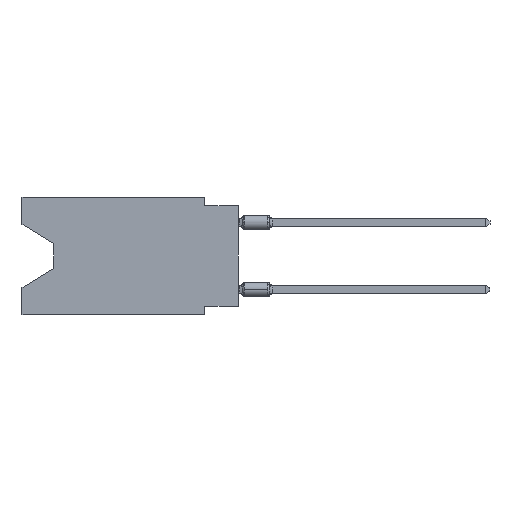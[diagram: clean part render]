
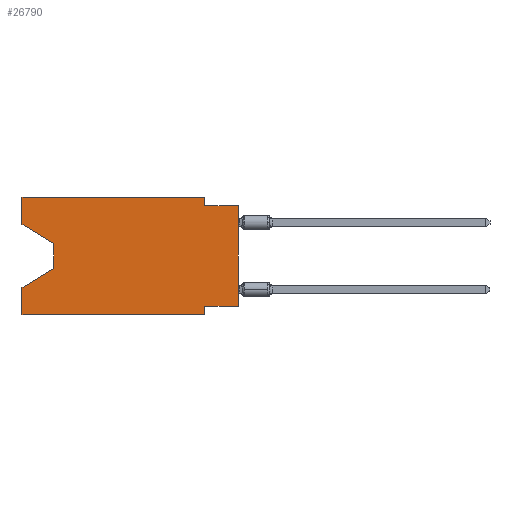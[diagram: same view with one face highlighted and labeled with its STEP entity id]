
A CAD part, left-side view. The second image highlights one B-rep face of the part: STEP entity #26790.
In plain terms, the highlighted planar face has unit normal (-1, 0, 0).
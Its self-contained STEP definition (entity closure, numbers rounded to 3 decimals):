
#3 = VECTOR ( 'NONE', #8153, 1000. ) ;
#32 = DIRECTION ( 'NONE',  ( 0., -1., 0. ) ) ;
#323 = VERTEX_POINT ( 'NONE', #29746 ) ;
#369 = LINE ( 'NONE', #28039, #20729 ) ;
#411 = DIRECTION ( 'NONE',  ( 0., 0., 1. ) ) ;
#494 = VECTOR ( 'NONE', #32, 1000. ) ;
#666 = CARTESIAN_POINT ( 'NONE',  ( 0., 16.383, 0. ) ) ;
#976 = DIRECTION ( 'NONE',  ( 0., 0., 1. ) ) ;
#1653 = EDGE_CURVE ( 'NONE', #4781, #33622, #13022, .T. ) ;
#1705 = VERTEX_POINT ( 'NONE', #1808 ) ;
#1808 = CARTESIAN_POINT ( 'NONE',  ( 0., 16.383, -2.038 ) ) ;
#1922 = VECTOR ( 'NONE', #24212, 1000. ) ;
#2004 = EDGE_CURVE ( 'NONE', #2498, #8590, #10922, .T. ) ;
#2134 = EDGE_CURVE ( 'NONE', #1705, #15088, #6054, .T. ) ;
#2196 = VERTEX_POINT ( 'NONE', #30822 ) ;
#2271 = CARTESIAN_POINT ( 'NONE',  ( 0., 2.54, 0. ) ) ;
#2498 = VERTEX_POINT ( 'NONE', #13072 ) ;
#2718 = CARTESIAN_POINT ( 'NONE',  ( 0., 16.383, -8.89 ) ) ;
#2837 = DIRECTION ( 'NONE',  ( 0., 0., -1. ) ) ;
#2867 = VECTOR ( 'NONE', #18896, 1000. ) ;
#3170 = EDGE_CURVE ( 'NONE', #2196, #8590, #26371, .T. ) ;
#3635 = DIRECTION ( 'NONE',  ( 0., 0., -1. ) ) ;
#3672 = EDGE_CURVE ( 'NONE', #15088, #33728, #13118, .T. ) ;
#3768 = ORIENTED_EDGE ( 'NONE', *, *, #2004, .T. ) ;
#3801 = CARTESIAN_POINT ( 'NONE',  ( 0., 16.383, 0. ) ) ;
#4375 = CARTESIAN_POINT ( 'NONE',  ( 0., 13.97, -3.505 ) ) ;
#4781 = VERTEX_POINT ( 'NONE', #31938 ) ;
#6054 = LINE ( 'NONE', #6597, #19264 ) ;
#6102 = CARTESIAN_POINT ( 'NONE',  ( 0., 2.54, 0. ) ) ;
#6143 = ORIENTED_EDGE ( 'NONE', *, *, #29639, .F. ) ;
#6597 = CARTESIAN_POINT ( 'NONE',  ( 0., 16.383, 0. ) ) ;
#6748 = CARTESIAN_POINT ( 'NONE',  ( 0., 16.383, -6.852 ) ) ;
#6887 = ORIENTED_EDGE ( 'NONE', *, *, #19787, .F. ) ;
#7578 = EDGE_CURVE ( 'NONE', #31840, #2498, #369, .T. ) ;
#7704 = CARTESIAN_POINT ( 'NONE',  ( 0., 16.383, 0. ) ) ;
#7708 = CARTESIAN_POINT ( 'NONE',  ( 0., 0., -8.255 ) ) ;
#7753 = LINE ( 'NONE', #30144, #22326 ) ;
#7934 = ORIENTED_EDGE ( 'NONE', *, *, #1653, .F. ) ;
#8043 = DIRECTION ( 'NONE',  ( 0., 0.855, -0.519 ) ) ;
#8153 = DIRECTION ( 'NONE',  ( 0., -1., 0. ) ) ;
#8253 = ORIENTED_EDGE ( 'NONE', *, *, #31693, .T. ) ;
#8590 = VERTEX_POINT ( 'NONE', #6748 ) ;
#9278 = CARTESIAN_POINT ( 'NONE',  ( 0., 0., 0. ) ) ;
#10867 = EDGE_CURVE ( 'NONE', #20718, #18394, #35172, .T. ) ;
#10922 = LINE ( 'NONE', #27208, #11189 ) ;
#11189 = VECTOR ( 'NONE', #8043, 1000. ) ;
#11339 = PLANE ( 'NONE',  #31923 ) ;
#11459 = VECTOR ( 'NONE', #26016, 1000. ) ;
#13022 = LINE ( 'NONE', #21503, #1922 ) ;
#13072 = CARTESIAN_POINT ( 'NONE',  ( 0., 13.97, -5.385 ) ) ;
#13118 = LINE ( 'NONE', #7704, #494 ) ;
#13483 = ORIENTED_EDGE ( 'NONE', *, *, #24575, .T. ) ;
#14204 = EDGE_CURVE ( 'NONE', #1705, #31840, #7753, .T. ) ;
#14849 = ORIENTED_EDGE ( 'NONE', *, *, #2134, .F. ) ;
#15088 = VERTEX_POINT ( 'NONE', #3801 ) ;
#16767 = FACE_OUTER_BOUND ( 'NONE', #23823, .T. ) ;
#18394 = VERTEX_POINT ( 'NONE', #23117 ) ;
#18756 = ORIENTED_EDGE ( 'NONE', *, *, #3170, .F. ) ;
#18788 = ORIENTED_EDGE ( 'NONE', *, *, #7578, .T. ) ;
#18896 = DIRECTION ( 'NONE',  ( 0., 1., 0. ) ) ;
#19264 = VECTOR ( 'NONE', #976, 1000. ) ;
#19731 = CARTESIAN_POINT ( 'NONE',  ( 0., 2.54, -8.89 ) ) ;
#19787 = EDGE_CURVE ( 'NONE', #18394, #323, #33647, .T. ) ;
#20397 = ORIENTED_EDGE ( 'NONE', *, *, #14204, .T. ) ;
#20718 = VERTEX_POINT ( 'NONE', #35223 ) ;
#20729 = VECTOR ( 'NONE', #22437, 1000. ) ;
#21086 = ORIENTED_EDGE ( 'NONE', *, *, #3672, .F. ) ;
#21503 = CARTESIAN_POINT ( 'NONE',  ( 0., 0., -0.635 ) ) ;
#22326 = VECTOR ( 'NONE', #29792, 1000. ) ;
#22437 = DIRECTION ( 'NONE',  ( 0., 0., -1. ) ) ;
#22557 = DIRECTION ( 'NONE',  ( 1., 0., 0. ) ) ;
#22745 = DIRECTION ( 'NONE',  ( 0., 0., -1. ) ) ;
#22759 = CARTESIAN_POINT ( 'NONE',  ( 0., 0., -0.635 ) ) ;
#22816 = VECTOR ( 'NONE', #22745, 1000. ) ;
#22919 = LINE ( 'NONE', #6102, #22816 ) ;
#23117 = CARTESIAN_POINT ( 'NONE',  ( 0., 2.54, -8.255 ) ) ;
#23823 = EDGE_LOOP ( 'NONE', ( #20397, #18788, #3768, #18756, #13483, #6887, #31657, #8253, #7934, #6143, #21086, #14849 ) ) ;
#24212 = DIRECTION ( 'NONE',  ( 0., -1., 0. ) ) ;
#24575 = EDGE_CURVE ( 'NONE', #2196, #323, #32902, .T. ) ;
#26016 = DIRECTION ( 'NONE',  ( 0., 0., 1. ) ) ;
#26371 = LINE ( 'NONE', #31795, #11459 ) ;
#26790 = ADVANCED_FACE ( 'NONE', ( #16767 ), #11339, .F. ) ;
#27208 = CARTESIAN_POINT ( 'NONE',  ( 0., 13.97, -5.385 ) ) ;
#27521 = VECTOR ( 'NONE', #411, 1000. ) ;
#28039 = CARTESIAN_POINT ( 'NONE',  ( 0., 13.97, -3.505 ) ) ;
#28085 = LINE ( 'NONE', #9278, #27521 ) ;
#29639 = EDGE_CURVE ( 'NONE', #33728, #4781, #22919, .T. ) ;
#29746 = CARTESIAN_POINT ( 'NONE',  ( 0., 2.54, -8.89 ) ) ;
#29792 = DIRECTION ( 'NONE',  ( 0., -0.855, -0.519 ) ) ;
#30144 = CARTESIAN_POINT ( 'NONE',  ( 0., 16.383, -2.038 ) ) ;
#30822 = CARTESIAN_POINT ( 'NONE',  ( 0., 16.383, -8.89 ) ) ;
#31657 = ORIENTED_EDGE ( 'NONE', *, *, #10867, .F. ) ;
#31693 = EDGE_CURVE ( 'NONE', #20718, #33622, #28085, .T. ) ;
#31795 = CARTESIAN_POINT ( 'NONE',  ( 0., 16.383, 0. ) ) ;
#31840 = VERTEX_POINT ( 'NONE', #4375 ) ;
#31923 = AXIS2_PLACEMENT_3D ( 'NONE', #666, #22557, #2837 ) ;
#31938 = CARTESIAN_POINT ( 'NONE',  ( 0., 2.54, -0.635 ) ) ;
#32902 = LINE ( 'NONE', #2718, #3 ) ;
#33622 = VERTEX_POINT ( 'NONE', #22759 ) ;
#33647 = LINE ( 'NONE', #19731, #34096 ) ;
#33728 = VERTEX_POINT ( 'NONE', #2271 ) ;
#34096 = VECTOR ( 'NONE', #3635, 1000. ) ;
#35172 = LINE ( 'NONE', #7708, #2867 ) ;
#35223 = CARTESIAN_POINT ( 'NONE',  ( 0., 0., -8.255 ) ) ;
